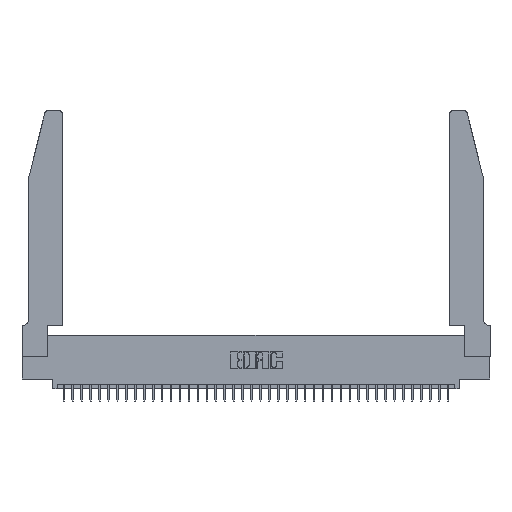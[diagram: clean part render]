
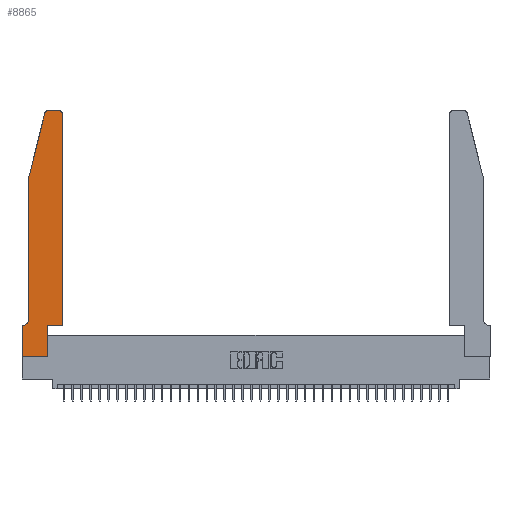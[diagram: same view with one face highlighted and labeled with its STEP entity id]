
A CAD part, top view. The second image highlights one B-rep face of the part: STEP entity #8865.
In plain terms, the highlighted planar face has unit normal (0, 0, 1).
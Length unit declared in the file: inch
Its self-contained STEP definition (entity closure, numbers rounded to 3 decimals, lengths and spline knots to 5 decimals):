
#29 = ORIENTED_EDGE ( 'NONE', *, *, #18031, .T. ) ;
#336 = ORIENTED_EDGE ( 'NONE', *, *, #10218, .T. ) ;
#381 = CARTESIAN_POINT ( 'NONE',  ( 0.4205, 2.75, 0.37 ) ) ;
#721 = DIRECTION ( 'NONE',  ( -1., 0., 0. ) ) ;
#1299 = EDGE_CURVE ( 'NONE', #7906, #33266, #35003, .T. ) ;
#1705 = EDGE_CURVE ( 'NONE', #31809, #35323, #8879, .T. ) ;
#1781 = CARTESIAN_POINT ( 'NONE',  ( 0., 0.35, 0.37 ) ) ;
#1844 = AXIS2_PLACEMENT_3D ( 'NONE', #3687, #15987, #31479 ) ;
#2446 = VECTOR ( 'NONE', #27643, 39.37008 ) ;
#2870 = ORIENTED_EDGE ( 'NONE', *, *, #20938, .T. ) ;
#3687 = CARTESIAN_POINT ( 'NONE',  ( 0.4205, 2.72, 0.37 ) ) ;
#4308 = CARTESIAN_POINT ( 'NONE',  ( 0.2865, 0.35, 0.37 ) ) ;
#4396 = DIRECTION ( 'NONE',  ( 0., 0., 1. ) ) ;
#4421 = ORIENTED_EDGE ( 'NONE', *, *, #10479, .T. ) ;
#4931 = CIRCLE ( 'NONE', #1844, 0.03 ) ;
#5949 = CARTESIAN_POINT ( 'NONE',  ( 0.0055, 0.42, 0.37 ) ) ;
#6066 = VERTEX_POINT ( 'NONE', #381 ) ;
#6075 = LINE ( 'NONE', #24750, #8604 ) ;
#6579 = LINE ( 'NONE', #15319, #21159 ) ;
#7156 = EDGE_CURVE ( 'NONE', #10198, #8818, #27734, .T. ) ;
#7475 = CARTESIAN_POINT ( 'NONE',  ( 0., 0., 0.37 ) ) ;
#7564 = PLANE ( 'NONE',  #39233 ) ;
#7906 = VERTEX_POINT ( 'NONE', #25156 ) ;
#8037 = EDGE_CURVE ( 'NONE', #35323, #9069, #32677, .T. ) ;
#8047 = CARTESIAN_POINT ( 'NONE',  ( 0.4505, 0.35, 0.37 ) ) ;
#8604 = VECTOR ( 'NONE', #721, 39.37008 ) ;
#8818 = VERTEX_POINT ( 'NONE', #13326 ) ;
#8865 = ADVANCED_FACE ( 'NONE', ( #16124 ), #7564, .T. ) ;
#8879 = LINE ( 'NONE', #33116, #22975 ) ;
#9069 = VERTEX_POINT ( 'NONE', #21244 ) ;
#10198 = VERTEX_POINT ( 'NONE', #15901 ) ;
#10218 = EDGE_CURVE ( 'NONE', #38796, #31818, #22789, .T. ) ;
#10226 = LINE ( 'NONE', #22339, #13274 ) ;
#10479 = EDGE_CURVE ( 'NONE', #6066, #10198, #6075, .T. ) ;
#10586 = AXIS2_PLACEMENT_3D ( 'NONE', #31066, #16354, #12980 ) ;
#10862 = CARTESIAN_POINT ( 'NONE',  ( 0., 0., 0.37 ) ) ;
#11549 = ORIENTED_EDGE ( 'NONE', *, *, #17556, .T. ) ;
#12822 = EDGE_CURVE ( 'NONE', #31818, #22450, #6579, .T. ) ;
#12980 = DIRECTION ( 'NONE',  ( 1., 0., 0. ) ) ;
#13274 = VECTOR ( 'NONE', #34470, 39.37008 ) ;
#13326 = CARTESIAN_POINT ( 'NONE',  ( 0.25487, 2.72718, 0.37 ) ) ;
#15113 = VECTOR ( 'NONE', #38435, 39.37008 ) ;
#15312 = ORIENTED_EDGE ( 'NONE', *, *, #1299, .T. ) ;
#15319 = CARTESIAN_POINT ( 'NONE',  ( 0., 0., 0.37 ) ) ;
#15901 = CARTESIAN_POINT ( 'NONE',  ( 0.284, 2.75, 0.37 ) ) ;
#15987 = DIRECTION ( 'NONE',  ( 0., 0., 1. ) ) ;
#16013 = VECTOR ( 'NONE', #19487, 39.37008 ) ;
#16124 = FACE_OUTER_BOUND ( 'NONE', #32261, .T. ) ;
#16354 = DIRECTION ( 'NONE',  ( 0., 0., 1. ) ) ;
#16899 = CARTESIAN_POINT ( 'NONE',  ( 0.2865, 0.35, 0.37 ) ) ;
#17014 = CARTESIAN_POINT ( 'NONE',  ( 0.0055, 0.35, 0.37 ) ) ;
#17476 = ORIENTED_EDGE ( 'NONE', *, *, #1705, .T. ) ;
#17490 = EDGE_CURVE ( 'NONE', #9069, #6066, #4931, .T. ) ;
#17556 = EDGE_CURVE ( 'NONE', #20173, #7906, #10226, .T. ) ;
#17865 = AXIS2_PLACEMENT_3D ( 'NONE', #5949, #17870, #30201 ) ;
#17870 = DIRECTION ( 'NONE',  ( 0., 0., -1. ) ) ;
#18031 = EDGE_CURVE ( 'NONE', #22450, #31809, #22473, .T. ) ;
#18301 = DIRECTION ( 'NONE',  ( 1., 0., 0. ) ) ;
#19020 = CARTESIAN_POINT ( 'NONE',  ( 0.0755, 2., 0.37 ) ) ;
#19487 = DIRECTION ( 'NONE',  ( 0., 1., 0. ) ) ;
#20173 = VERTEX_POINT ( 'NONE', #19020 ) ;
#20295 = ORIENTED_EDGE ( 'NONE', *, *, #22605, .T. ) ;
#20938 = EDGE_CURVE ( 'NONE', #8818, #20173, #29674, .T. ) ;
#21159 = VECTOR ( 'NONE', #18301, 39.37008 ) ;
#21244 = CARTESIAN_POINT ( 'NONE',  ( 0.4505, 2.72, 0.37 ) ) ;
#22339 = CARTESIAN_POINT ( 'NONE',  ( 0.0755, 2., 0.37 ) ) ;
#22450 = VERTEX_POINT ( 'NONE', #23621 ) ;
#22473 = LINE ( 'NONE', #16899, #16013 ) ;
#22605 = EDGE_CURVE ( 'NONE', #33266, #38796, #25530, .T. ) ;
#22789 = LINE ( 'NONE', #10862, #2446 ) ;
#22975 = VECTOR ( 'NONE', #23400, 39.37008 ) ;
#23400 = DIRECTION ( 'NONE',  ( 1., 0., 0. ) ) ;
#23621 = CARTESIAN_POINT ( 'NONE',  ( 0.2865, 0., 0.37 ) ) ;
#24750 = CARTESIAN_POINT ( 'NONE',  ( 0.2605, 2.75, 0.37 ) ) ;
#24935 = CARTESIAN_POINT ( 'NONE',  ( 0.0755, 0.35, 0.37 ) ) ;
#25156 = CARTESIAN_POINT ( 'NONE',  ( 0.0755, 0.42, 0.37 ) ) ;
#25258 = DIRECTION ( 'NONE',  ( 1., 0., 0. ) ) ;
#25530 = LINE ( 'NONE', #24935, #28512 ) ;
#25858 = VECTOR ( 'NONE', #39053, 39.37008 ) ;
#26326 = CARTESIAN_POINT ( 'NONE',  ( 0.0755, 2., 0.37 ) ) ;
#26837 = ORIENTED_EDGE ( 'NONE', *, *, #17490, .T. ) ;
#27178 = ORIENTED_EDGE ( 'NONE', *, *, #7156, .T. ) ;
#27643 = DIRECTION ( 'NONE',  ( 0., -1., 0. ) ) ;
#27734 = CIRCLE ( 'NONE', #10586, 0.03 ) ;
#28247 = CARTESIAN_POINT ( 'NONE',  ( 0., 0.35, 0.37 ) ) ;
#28512 = VECTOR ( 'NONE', #28899, 39.37008 ) ;
#28899 = DIRECTION ( 'NONE',  ( -1., 0., 0. ) ) ;
#29674 = LINE ( 'NONE', #26326, #15113 ) ;
#30201 = DIRECTION ( 'NONE',  ( -1., 0., 0. ) ) ;
#31066 = CARTESIAN_POINT ( 'NONE',  ( 0.284, 2.72, 0.37 ) ) ;
#31479 = DIRECTION ( 'NONE',  ( 1., 0., 0. ) ) ;
#31809 = VERTEX_POINT ( 'NONE', #4308 ) ;
#31818 = VERTEX_POINT ( 'NONE', #7475 ) ;
#31838 = CARTESIAN_POINT ( 'NONE',  ( 0.4505, 0.35, 0.37 ) ) ;
#32261 = EDGE_LOOP ( 'NONE', ( #4421, #27178, #2870, #11549, #15312, #20295, #336, #39219, #29, #17476, #35022, #26837 ) ) ;
#32677 = LINE ( 'NONE', #8047, #25858 ) ;
#33116 = CARTESIAN_POINT ( 'NONE',  ( 0.4505, 0.35, 0.37 ) ) ;
#33266 = VERTEX_POINT ( 'NONE', #17014 ) ;
#34470 = DIRECTION ( 'NONE',  ( 0., -1., 0. ) ) ;
#35003 = CIRCLE ( 'NONE', #17865, 0.07 ) ;
#35022 = ORIENTED_EDGE ( 'NONE', *, *, #8037, .T. ) ;
#35323 = VERTEX_POINT ( 'NONE', #31838 ) ;
#38435 = DIRECTION ( 'NONE',  ( -0.239, -0.971, 0. ) ) ;
#38796 = VERTEX_POINT ( 'NONE', #1781 ) ;
#39053 = DIRECTION ( 'NONE',  ( 0., 1., 0. ) ) ;
#39219 = ORIENTED_EDGE ( 'NONE', *, *, #12822, .T. ) ;
#39233 = AXIS2_PLACEMENT_3D ( 'NONE', #28247, #4396, #25258 ) ;
